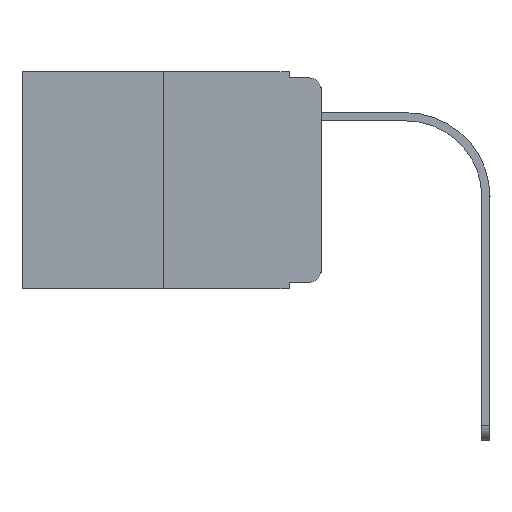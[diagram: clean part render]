
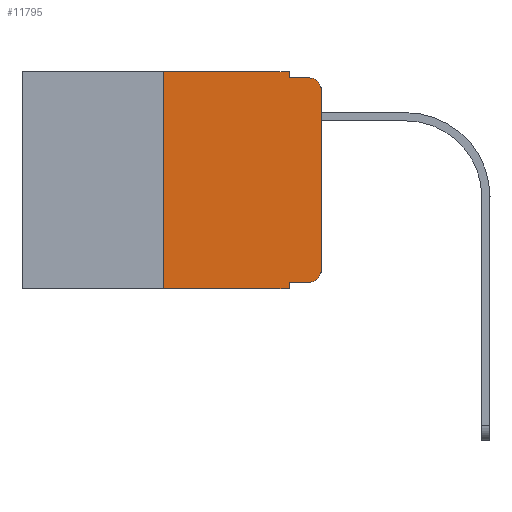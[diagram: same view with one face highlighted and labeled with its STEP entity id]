
A CAD part, left-side view. The second image highlights one B-rep face of the part: STEP entity #11795.
In plain terms, the highlighted planar face has unit normal (-1, 0, 0).
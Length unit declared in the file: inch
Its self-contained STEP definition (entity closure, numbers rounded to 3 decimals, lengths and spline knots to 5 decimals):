
#118 = VECTOR ( 'NONE', #8173, 39.37008 ) ;
#159 = ORIENTED_EDGE ( 'NONE', *, *, #2715, .F. ) ;
#334 = CARTESIAN_POINT ( 'NONE',  ( 0., 0.25, 0. ) ) ;
#495 = DIRECTION ( 'NONE',  ( 0., 0., -1. ) ) ;
#593 = LINE ( 'NONE', #9433, #18094 ) ;
#717 = EDGE_CURVE ( 'NONE', #5833, #10014, #5476, .T. ) ;
#1498 = VECTOR ( 'NONE', #13258, 39.37008 ) ;
#2003 = EDGE_CURVE ( 'NONE', #6497, #8423, #593, .T. ) ;
#2006 = CIRCLE ( 'NONE', #12141, 0.02 ) ;
#2599 = LINE ( 'NONE', #17094, #118 ) ;
#2715 = EDGE_CURVE ( 'NONE', #8423, #12175, #7008, .T. ) ;
#3070 = CARTESIAN_POINT ( 'NONE',  ( 0., 0., 0. ) ) ;
#3221 = ORIENTED_EDGE ( 'NONE', *, *, #17466, .T. ) ;
#3716 = CARTESIAN_POINT ( 'NONE',  ( 0., 0.473, 0. ) ) ;
#4210 = EDGE_CURVE ( 'NONE', #5027, #7295, #8288, .T. ) ;
#4346 = VECTOR ( 'NONE', #11276, 39.37008 ) ;
#4699 = LINE ( 'NONE', #3070, #1498 ) ;
#5027 = VERTEX_POINT ( 'NONE', #13397 ) ;
#5119 = DIRECTION ( 'NONE',  ( 0., 0., -1. ) ) ;
#5299 = DIRECTION ( 'NONE',  ( 0., 0., 1. ) ) ;
#5397 = ORIENTED_EDGE ( 'NONE', *, *, #4210, .F. ) ;
#5476 = CIRCLE ( 'NONE', #10365, 0.02 ) ;
#5662 = VECTOR ( 'NONE', #6274, 39.37008 ) ;
#5675 = VERTEX_POINT ( 'NONE', #17189 ) ;
#5833 = VERTEX_POINT ( 'NONE', #13076 ) ;
#6274 = DIRECTION ( 'NONE',  ( 0., -1., 0. ) ) ;
#6497 = VERTEX_POINT ( 'NONE', #13423 ) ;
#6684 = VECTOR ( 'NONE', #11571, 39.37008 ) ;
#6863 = CARTESIAN_POINT ( 'NONE',  ( 0., 0.051, -0.01 ) ) ;
#7008 = LINE ( 'NONE', #17166, #11704 ) ;
#7295 = VERTEX_POINT ( 'NONE', #12197 ) ;
#7640 = EDGE_CURVE ( 'NONE', #10014, #9695, #4699, .T. ) ;
#7693 = LINE ( 'NONE', #15458, #5662 ) ;
#8173 = DIRECTION ( 'NONE',  ( 0., 0., -1. ) ) ;
#8288 = LINE ( 'NONE', #6863, #4346 ) ;
#8423 = VERTEX_POINT ( 'NONE', #334 ) ;
#8462 = VECTOR ( 'NONE', #10551, 39.37008 ) ;
#8476 = ORIENTED_EDGE ( 'NONE', *, *, #15400, .T. ) ;
#8589 = CARTESIAN_POINT ( 'NONE',  ( 0., 0., -0.313 ) ) ;
#9308 = ORIENTED_EDGE ( 'NONE', *, *, #717, .T. ) ;
#9433 = CARTESIAN_POINT ( 'NONE',  ( 0., 0.25, 0. ) ) ;
#9435 = ORIENTED_EDGE ( 'NONE', *, *, #14114, .T. ) ;
#9695 = VERTEX_POINT ( 'NONE', #17254 ) ;
#10014 = VERTEX_POINT ( 'NONE', #8589 ) ;
#10365 = AXIS2_PLACEMENT_3D ( 'NONE', #15102, #13943, #495 ) ;
#10551 = DIRECTION ( 'NONE',  ( 0., 0., -1. ) ) ;
#10911 = EDGE_CURVE ( 'NONE', #12175, #5027, #2599, .T. ) ;
#11010 = CARTESIAN_POINT ( 'NONE',  ( 0., 0.051, 0. ) ) ;
#11028 = FACE_OUTER_BOUND ( 'NONE', #15592, .T. ) ;
#11276 = DIRECTION ( 'NONE',  ( 0., -1., 0. ) ) ;
#11455 = VERTEX_POINT ( 'NONE', #11763 ) ;
#11571 = DIRECTION ( 'NONE',  ( 0., -1., 0. ) ) ;
#11704 = VECTOR ( 'NONE', #12860, 39.37008 ) ;
#11763 = CARTESIAN_POINT ( 'NONE',  ( 0., 0.051, -0.333 ) ) ;
#11795 = ADVANCED_FACE ( 'NONE', ( #11028 ), #16862, .F. ) ;
#11799 = CARTESIAN_POINT ( 'NONE',  ( 0., 0.051, 0. ) ) ;
#11985 = LINE ( 'NONE', #11799, #8462 ) ;
#12141 = AXIS2_PLACEMENT_3D ( 'NONE', #13671, #15307, #5119 ) ;
#12175 = VERTEX_POINT ( 'NONE', #11010 ) ;
#12197 = CARTESIAN_POINT ( 'NONE',  ( 0., 0.02, -0.01 ) ) ;
#12609 = ORIENTED_EDGE ( 'NONE', *, *, #2003, .F. ) ;
#12852 = DIRECTION ( 'NONE',  ( 1., 0., 0. ) ) ;
#12860 = DIRECTION ( 'NONE',  ( 0., -1., 0. ) ) ;
#13013 = LINE ( 'NONE', #17597, #6684 ) ;
#13076 = CARTESIAN_POINT ( 'NONE',  ( 0., 0.02, -0.333 ) ) ;
#13258 = DIRECTION ( 'NONE',  ( 0., 0., 1. ) ) ;
#13397 = CARTESIAN_POINT ( 'NONE',  ( 0., 0.051, -0.01 ) ) ;
#13423 = CARTESIAN_POINT ( 'NONE',  ( 0., 0.25, -0.343 ) ) ;
#13646 = AXIS2_PLACEMENT_3D ( 'NONE', #3716, #12852, #14098 ) ;
#13671 = CARTESIAN_POINT ( 'NONE',  ( 0., 0.02, -0.03 ) ) ;
#13943 = DIRECTION ( 'NONE',  ( -1., 0., 0. ) ) ;
#14098 = DIRECTION ( 'NONE',  ( 0., 0., -1. ) ) ;
#14114 = EDGE_CURVE ( 'NONE', #6497, #5675, #7693, .T. ) ;
#15102 = CARTESIAN_POINT ( 'NONE',  ( 0., 0.02, -0.313 ) ) ;
#15307 = DIRECTION ( 'NONE',  ( -1., 0., 0. ) ) ;
#15400 = EDGE_CURVE ( 'NONE', #9695, #7295, #2006, .T. ) ;
#15425 = ORIENTED_EDGE ( 'NONE', *, *, #7640, .T. ) ;
#15458 = CARTESIAN_POINT ( 'NONE',  ( 0., 0.473, -0.343 ) ) ;
#15543 = EDGE_CURVE ( 'NONE', #11455, #5675, #11985, .T. ) ;
#15592 = EDGE_LOOP ( 'NONE', ( #15425, #8476, #5397, #18292, #159, #12609, #9435, #18617, #3221, #9308 ) ) ;
#16862 = PLANE ( 'NONE',  #13646 ) ;
#17094 = CARTESIAN_POINT ( 'NONE',  ( 0., 0.051, 0. ) ) ;
#17166 = CARTESIAN_POINT ( 'NONE',  ( 0., 0.473, 0. ) ) ;
#17189 = CARTESIAN_POINT ( 'NONE',  ( 0., 0.051, -0.343 ) ) ;
#17254 = CARTESIAN_POINT ( 'NONE',  ( 0., 0., -0.03 ) ) ;
#17466 = EDGE_CURVE ( 'NONE', #11455, #5833, #13013, .T. ) ;
#17597 = CARTESIAN_POINT ( 'NONE',  ( 0., 0.051, -0.333 ) ) ;
#18094 = VECTOR ( 'NONE', #5299, 39.37008 ) ;
#18292 = ORIENTED_EDGE ( 'NONE', *, *, #10911, .F. ) ;
#18617 = ORIENTED_EDGE ( 'NONE', *, *, #15543, .F. ) ;
